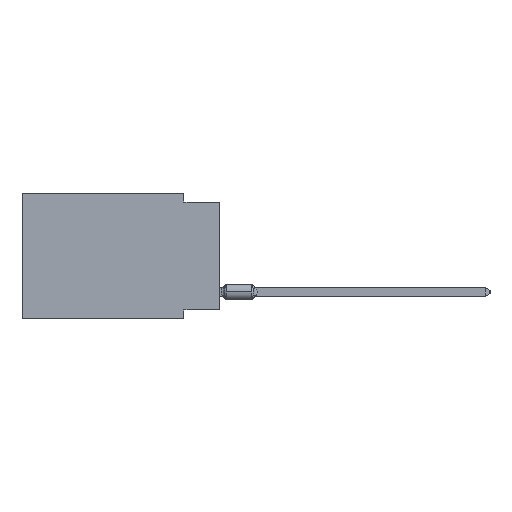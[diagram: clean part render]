
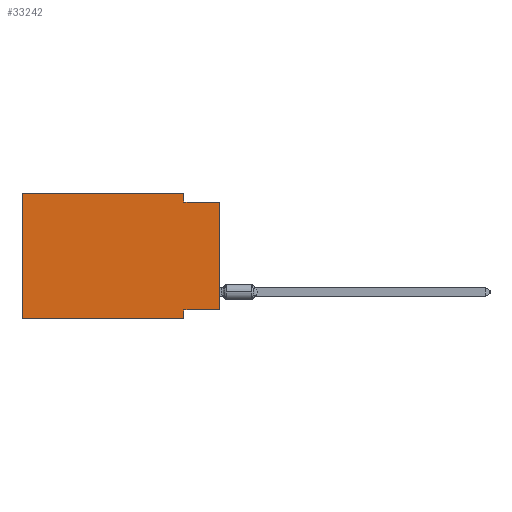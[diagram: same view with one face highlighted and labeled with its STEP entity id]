
A CAD part, left-side view. The second image highlights one B-rep face of the part: STEP entity #33242.
In plain terms, the highlighted planar face has unit normal (-1, 0, 0).
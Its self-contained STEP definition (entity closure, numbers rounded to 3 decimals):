
#827 = CARTESIAN_POINT ( 'NONE',  ( 0., 13.97, 0. ) ) ;
#1377 = CARTESIAN_POINT ( 'NONE',  ( 0., 2.54, -8.89 ) ) ;
#3274 = VECTOR ( 'NONE', #34111, 1000. ) ;
#3375 = VERTEX_POINT ( 'NONE', #38075 ) ;
#5003 = VERTEX_POINT ( 'NONE', #61102 ) ;
#7252 = EDGE_CURVE ( 'NONE', #5003, #37636, #29169, .T. ) ;
#7895 = EDGE_LOOP ( 'NONE', ( #53670, #69041, #53219, #52105, #10512, #28161, #68842, #9859 ) ) ;
#9859 = ORIENTED_EDGE ( 'NONE', *, *, #20862, .F. ) ;
#10186 = VECTOR ( 'NONE', #35084, 1000. ) ;
#10512 = ORIENTED_EDGE ( 'NONE', *, *, #7252, .F. ) ;
#11549 = CARTESIAN_POINT ( 'NONE',  ( 0., 2.54, -8.89 ) ) ;
#13925 = VERTEX_POINT ( 'NONE', #25044 ) ;
#13979 = AXIS2_PLACEMENT_3D ( 'NONE', #27269, #56338, #16772 ) ;
#14406 = EDGE_CURVE ( 'NONE', #59394, #3375, #35049, .T. ) ;
#16772 = DIRECTION ( 'NONE',  ( 0., 0., -1. ) ) ;
#17149 = DIRECTION ( 'NONE',  ( 0., -1., 0. ) ) ;
#20862 = EDGE_CURVE ( 'NONE', #59394, #58696, #36077, .T. ) ;
#21309 = FACE_OUTER_BOUND ( 'NONE', #7895, .T. ) ;
#24638 = LINE ( 'NONE', #63456, #58700 ) ;
#25044 = CARTESIAN_POINT ( 'NONE',  ( 0., 2.54, -0.635 ) ) ;
#25981 = CARTESIAN_POINT ( 'NONE',  ( 0., 0., -8.255 ) ) ;
#27205 = CARTESIAN_POINT ( 'NONE',  ( 0., 2.54, -8.255 ) ) ;
#27269 = CARTESIAN_POINT ( 'NONE',  ( 0., 13.97, 0. ) ) ;
#28161 = ORIENTED_EDGE ( 'NONE', *, *, #36510, .T. ) ;
#28193 = VECTOR ( 'NONE', #46627, 1000. ) ;
#29169 = LINE ( 'NONE', #62379, #30229 ) ;
#29835 = CARTESIAN_POINT ( 'NONE',  ( 0., 0., 0. ) ) ;
#29858 = LINE ( 'NONE', #68679, #28193 ) ;
#30229 = VECTOR ( 'NONE', #56773, 1000. ) ;
#30444 = CARTESIAN_POINT ( 'NONE',  ( 0., 0., -8.255 ) ) ;
#33242 = ADVANCED_FACE ( 'NONE', ( #21309 ), #38822, .F. ) ;
#33460 = EDGE_CURVE ( 'NONE', #37636, #67580, #29858, .T. ) ;
#34111 = DIRECTION ( 'NONE',  ( 0., 0., -1. ) ) ;
#34347 = VECTOR ( 'NONE', #52581, 1000. ) ;
#34478 = CARTESIAN_POINT ( 'NONE',  ( 0., 2.54, 0. ) ) ;
#35049 = LINE ( 'NONE', #29835, #34347 ) ;
#35084 = DIRECTION ( 'NONE',  ( 0., 0., -1. ) ) ;
#36077 = LINE ( 'NONE', #25981, #60228 ) ;
#36510 = EDGE_CURVE ( 'NONE', #5003, #68469, #50389, .T. ) ;
#37636 = VERTEX_POINT ( 'NONE', #827 ) ;
#38075 = CARTESIAN_POINT ( 'NONE',  ( 0., 0., -0.635 ) ) ;
#38822 = PLANE ( 'NONE',  #13979 ) ;
#38830 = CARTESIAN_POINT ( 'NONE',  ( 0., 13.97, -8.89 ) ) ;
#41749 = VECTOR ( 'NONE', #17149, 1000. ) ;
#46627 = DIRECTION ( 'NONE',  ( 0., -1., 0. ) ) ;
#50389 = LINE ( 'NONE', #38830, #41749 ) ;
#51574 = CARTESIAN_POINT ( 'NONE',  ( 0., 2.54, 0. ) ) ;
#51866 = LINE ( 'NONE', #11549, #10186 ) ;
#51888 = EDGE_CURVE ( 'NONE', #67580, #13925, #62104, .T. ) ;
#52105 = ORIENTED_EDGE ( 'NONE', *, *, #33460, .F. ) ;
#52581 = DIRECTION ( 'NONE',  ( 0., 0., 1. ) ) ;
#53219 = ORIENTED_EDGE ( 'NONE', *, *, #51888, .F. ) ;
#53670 = ORIENTED_EDGE ( 'NONE', *, *, #14406, .T. ) ;
#56338 = DIRECTION ( 'NONE',  ( 1., 0., 0. ) ) ;
#56773 = DIRECTION ( 'NONE',  ( 0., 0., 1. ) ) ;
#57271 = EDGE_CURVE ( 'NONE', #13925, #3375, #24638, .T. ) ;
#58602 = DIRECTION ( 'NONE',  ( 0., -1., 0. ) ) ;
#58696 = VERTEX_POINT ( 'NONE', #27205 ) ;
#58700 = VECTOR ( 'NONE', #58602, 1000. ) ;
#58851 = DIRECTION ( 'NONE',  ( 0., 1., 0. ) ) ;
#59394 = VERTEX_POINT ( 'NONE', #30444 ) ;
#60228 = VECTOR ( 'NONE', #58851, 1000. ) ;
#61102 = CARTESIAN_POINT ( 'NONE',  ( 0., 13.97, -8.89 ) ) ;
#62104 = LINE ( 'NONE', #34478, #3274 ) ;
#62379 = CARTESIAN_POINT ( 'NONE',  ( 0., 13.97, 0. ) ) ;
#63456 = CARTESIAN_POINT ( 'NONE',  ( 0., 0., -0.635 ) ) ;
#67580 = VERTEX_POINT ( 'NONE', #51574 ) ;
#68469 = VERTEX_POINT ( 'NONE', #1377 ) ;
#68679 = CARTESIAN_POINT ( 'NONE',  ( 0., 13.97, 0. ) ) ;
#68842 = ORIENTED_EDGE ( 'NONE', *, *, #69678, .F. ) ;
#69041 = ORIENTED_EDGE ( 'NONE', *, *, #57271, .F. ) ;
#69678 = EDGE_CURVE ( 'NONE', #58696, #68469, #51866, .T. ) ;
